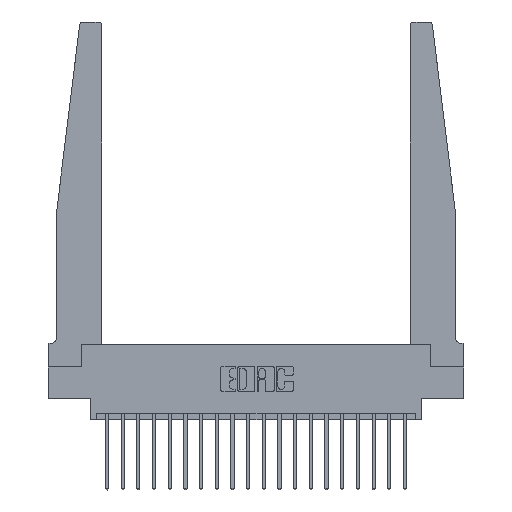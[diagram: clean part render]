
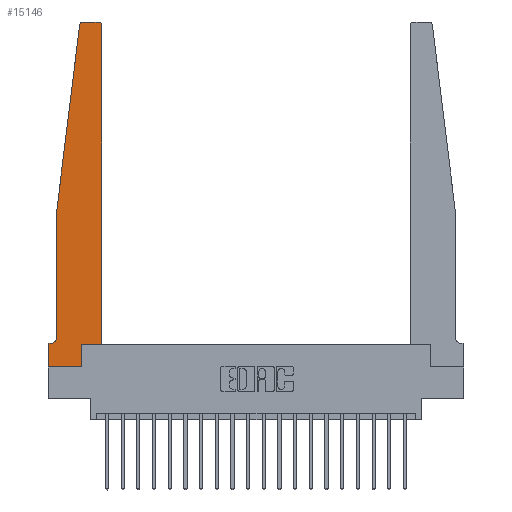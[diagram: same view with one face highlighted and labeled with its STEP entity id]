
A CAD part, top view. The second image highlights one B-rep face of the part: STEP entity #15146.
In plain terms, the highlighted planar face has unit normal (0, 0, 1).
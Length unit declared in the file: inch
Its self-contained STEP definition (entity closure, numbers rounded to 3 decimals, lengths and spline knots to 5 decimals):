
#378 = CARTESIAN_POINT ( 'NONE',  ( 0., 0., 0.37 ) ) ;
#545 = VECTOR ( 'NONE', #10814, 39.37008 ) ;
#699 = DIRECTION ( 'NONE',  ( 0., 0., -1. ) ) ;
#952 = LINE ( 'NONE', #4035, #1463 ) ;
#1463 = VECTOR ( 'NONE', #13651, 39.37008 ) ;
#1513 = LINE ( 'NONE', #378, #14876 ) ;
#1738 = DIRECTION ( 'NONE',  ( 0., 1., 0. ) ) ;
#1919 = VECTOR ( 'NONE', #11168, 39.37008 ) ;
#2298 = VERTEX_POINT ( 'NONE', #8453 ) ;
#2311 = CARTESIAN_POINT ( 'NONE',  ( 0.065, 0.1875, 0.37 ) ) ;
#2321 = CARTESIAN_POINT ( 'NONE',  ( 0., 0.1875, 0.37 ) ) ;
#2588 = VECTOR ( 'NONE', #1738, 39.37008 ) ;
#2607 = VECTOR ( 'NONE', #4593, 39.37008 ) ;
#2785 = CARTESIAN_POINT ( 'NONE',  ( 0.25, 2.75, 0.37 ) ) ;
#2881 = ORIENTED_EDGE ( 'NONE', *, *, #17257, .T. ) ;
#2905 = CARTESIAN_POINT ( 'NONE',  ( 0.395, 2.75, 0.37 ) ) ;
#3394 = CARTESIAN_POINT ( 'NONE',  ( 0.065, 1.25, 0.37 ) ) ;
#3942 = AXIS2_PLACEMENT_3D ( 'NONE', #5192, #16414, #6796 ) ;
#3977 = DIRECTION ( 'NONE',  ( -1., 0., 0. ) ) ;
#4026 = CARTESIAN_POINT ( 'NONE',  ( 0.065, 0.2375, 0.37 ) ) ;
#4035 = CARTESIAN_POINT ( 'NONE',  ( 0.2605, 0.18, 0.37 ) ) ;
#4593 = DIRECTION ( 'NONE',  ( -0.122, -0.992, 0. ) ) ;
#5192 = CARTESIAN_POINT ( 'NONE',  ( 0.27653, 2.72, 0.37 ) ) ;
#5538 = VECTOR ( 'NONE', #3977, 39.37008 ) ;
#5599 = PLANE ( 'NONE',  #20624 ) ;
#6058 = AXIS2_PLACEMENT_3D ( 'NONE', #10364, #699, #11965 ) ;
#6265 = ORIENTED_EDGE ( 'NONE', *, *, #8081, .T. ) ;
#6567 = CARTESIAN_POINT ( 'NONE',  ( 0.425, 0.18, 0.37 ) ) ;
#6655 = CARTESIAN_POINT ( 'NONE',  ( 0.425, 0.18, 0.37 ) ) ;
#6796 = DIRECTION ( 'NONE',  ( 1., 0., 0. ) ) ;
#6896 = VERTEX_POINT ( 'NONE', #7767 ) ;
#7162 = EDGE_CURVE ( 'NONE', #12444, #2298, #1513, .T. ) ;
#7543 = CARTESIAN_POINT ( 'NONE',  ( 0.24675, 2.72367, 0.37 ) ) ;
#7767 = CARTESIAN_POINT ( 'NONE',  ( 0., 0.1875, 0.37 ) ) ;
#7815 = DIRECTION ( 'NONE',  ( 0., 0., 1. ) ) ;
#8014 = EDGE_CURVE ( 'NONE', #14998, #11502, #9585, .T. ) ;
#8081 = EDGE_CURVE ( 'NONE', #13282, #16140, #9077, .T. ) ;
#8233 = EDGE_CURVE ( 'NONE', #12996, #6896, #18402, .T. ) ;
#8310 = CARTESIAN_POINT ( 'NONE',  ( 0.015, 0.1875, 0.37 ) ) ;
#8453 = CARTESIAN_POINT ( 'NONE',  ( 0.2605, 0., 0.37 ) ) ;
#8522 = CIRCLE ( 'NONE', #10275, 0.03 ) ;
#8681 = CARTESIAN_POINT ( 'NONE',  ( 0., 0., 0.37 ) ) ;
#8846 = DIRECTION ( 'NONE',  ( 1., 0., 0. ) ) ;
#9028 = ORIENTED_EDGE ( 'NONE', *, *, #8233, .T. ) ;
#9071 = EDGE_CURVE ( 'NONE', #17877, #16874, #8522, .T. ) ;
#9077 = CIRCLE ( 'NONE', #3942, 0.03 ) ;
#9513 = ORIENTED_EDGE ( 'NONE', *, *, #12831, .T. ) ;
#9585 = LINE ( 'NONE', #6655, #10080 ) ;
#10071 = CARTESIAN_POINT ( 'NONE',  ( 0.425, 2.72, 0.37 ) ) ;
#10080 = VECTOR ( 'NONE', #17925, 39.37008 ) ;
#10275 = AXIS2_PLACEMENT_3D ( 'NONE', #17441, #7815, #19066 ) ;
#10364 = CARTESIAN_POINT ( 'NONE',  ( 0.015, 0.2375, 0.37 ) ) ;
#10683 = ORIENTED_EDGE ( 'NONE', *, *, #14399, .T. ) ;
#10814 = DIRECTION ( 'NONE',  ( -1., 0., 0. ) ) ;
#11004 = LINE ( 'NONE', #17603, #1919 ) ;
#11018 = ORIENTED_EDGE ( 'NONE', *, *, #7162, .T. ) ;
#11168 = DIRECTION ( 'NONE',  ( 0., -1., 0. ) ) ;
#11178 = LINE ( 'NONE', #15800, #2607 ) ;
#11502 = VERTEX_POINT ( 'NONE', #12636 ) ;
#11652 = DIRECTION ( 'NONE',  ( 1., 0., 0. ) ) ;
#11965 = DIRECTION ( 'NONE',  ( -1., 0., 0. ) ) ;
#12254 = VERTEX_POINT ( 'NONE', #3394 ) ;
#12444 = VERTEX_POINT ( 'NONE', #8681 ) ;
#12636 = CARTESIAN_POINT ( 'NONE',  ( 0.425, 0.18, 0.37 ) ) ;
#12831 = EDGE_CURVE ( 'NONE', #6896, #12444, #11004, .T. ) ;
#12996 = VERTEX_POINT ( 'NONE', #8310 ) ;
#13282 = VERTEX_POINT ( 'NONE', #17858 ) ;
#13414 = LINE ( 'NONE', #2785, #545 ) ;
#13635 = ORIENTED_EDGE ( 'NONE', *, *, #19553, .T. ) ;
#13651 = DIRECTION ( 'NONE',  ( 0., 1., 0. ) ) ;
#13725 = EDGE_CURVE ( 'NONE', #12254, #14163, #18051, .T. ) ;
#14163 = VERTEX_POINT ( 'NONE', #4026 ) ;
#14399 = EDGE_CURVE ( 'NONE', #16140, #12254, #11178, .T. ) ;
#14472 = ORIENTED_EDGE ( 'NONE', *, *, #9071, .T. ) ;
#14759 = ORIENTED_EDGE ( 'NONE', *, *, #15566, .T. ) ;
#14876 = VECTOR ( 'NONE', #11652, 39.37008 ) ;
#14998 = VERTEX_POINT ( 'NONE', #19479 ) ;
#15146 = ADVANCED_FACE ( 'NONE', ( #18778 ), #5599, .T. ) ;
#15566 = EDGE_CURVE ( 'NONE', #11502, #17877, #19766, .T. ) ;
#15613 = DIRECTION ( 'NONE',  ( 0., -1., 0. ) ) ;
#15626 = CIRCLE ( 'NONE', #6058, 0.05 ) ;
#15686 = CARTESIAN_POINT ( 'NONE',  ( 0.065, 1.25, 0.37 ) ) ;
#15800 = CARTESIAN_POINT ( 'NONE',  ( 0.065, 1.25, 0.37 ) ) ;
#16140 = VERTEX_POINT ( 'NONE', #7543 ) ;
#16189 = EDGE_CURVE ( 'NONE', #16874, #13282, #13414, .T. ) ;
#16414 = DIRECTION ( 'NONE',  ( 0., 0., 1. ) ) ;
#16874 = VERTEX_POINT ( 'NONE', #2905 ) ;
#17160 = EDGE_LOOP ( 'NONE', ( #17605, #6265, #10683, #19450, #2881, #9028, #9513, #11018, #13635, #18408, #14759, #14472 ) ) ;
#17257 = EDGE_CURVE ( 'NONE', #14163, #12996, #15626, .T. ) ;
#17441 = CARTESIAN_POINT ( 'NONE',  ( 0.395, 2.72, 0.37 ) ) ;
#17529 = VECTOR ( 'NONE', #15613, 39.37008 ) ;
#17603 = CARTESIAN_POINT ( 'NONE',  ( 0., 0., 0.37 ) ) ;
#17605 = ORIENTED_EDGE ( 'NONE', *, *, #16189, .T. ) ;
#17858 = CARTESIAN_POINT ( 'NONE',  ( 0.27653, 2.75, 0.37 ) ) ;
#17877 = VERTEX_POINT ( 'NONE', #10071 ) ;
#17925 = DIRECTION ( 'NONE',  ( 1., 0., 0. ) ) ;
#18051 = LINE ( 'NONE', #15686, #17529 ) ;
#18402 = LINE ( 'NONE', #2311, #5538 ) ;
#18408 = ORIENTED_EDGE ( 'NONE', *, *, #8014, .T. ) ;
#18496 = DIRECTION ( 'NONE',  ( 0., 0., 1. ) ) ;
#18778 = FACE_OUTER_BOUND ( 'NONE', #17160, .T. ) ;
#19066 = DIRECTION ( 'NONE',  ( 1., 0., 0. ) ) ;
#19450 = ORIENTED_EDGE ( 'NONE', *, *, #13725, .T. ) ;
#19479 = CARTESIAN_POINT ( 'NONE',  ( 0.2605, 0.18, 0.37 ) ) ;
#19553 = EDGE_CURVE ( 'NONE', #2298, #14998, #952, .T. ) ;
#19766 = LINE ( 'NONE', #6567, #2588 ) ;
#20624 = AXIS2_PLACEMENT_3D ( 'NONE', #2321, #18496, #8846 ) ;
